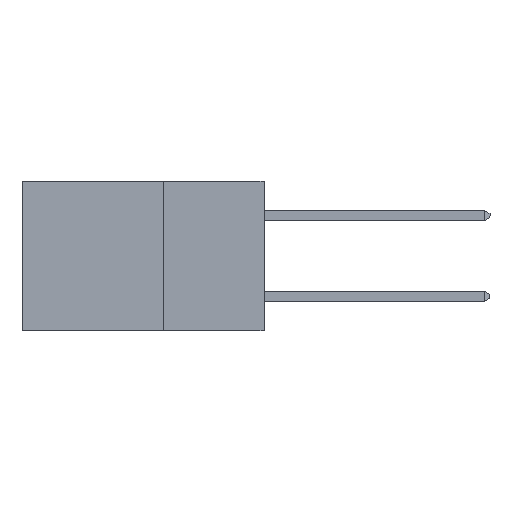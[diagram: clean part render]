
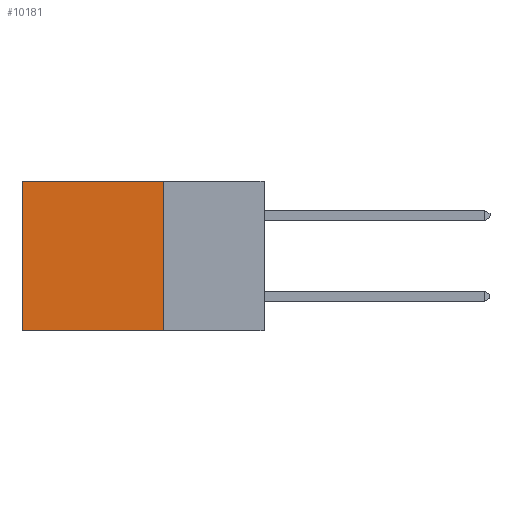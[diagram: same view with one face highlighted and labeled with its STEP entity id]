
A CAD part, left-side view. The second image highlights one B-rep face of the part: STEP entity #10181.
In plain terms, the highlighted planar face has unit normal (-1, 0, 0).
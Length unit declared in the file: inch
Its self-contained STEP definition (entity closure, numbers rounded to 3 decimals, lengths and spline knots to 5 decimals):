
#156 = CARTESIAN_POINT ( 'NONE',  ( 0.298, 0.25, 0. ) ) ;
#954 = VERTEX_POINT ( 'NONE', #5583 ) ;
#2154 = CARTESIAN_POINT ( 'NONE',  ( 0.298, 0.6, 0. ) ) ;
#3468 = EDGE_LOOP ( 'NONE', ( #4100, #5359, #7888, #10248 ) ) ;
#3909 = VERTEX_POINT ( 'NONE', #12758 ) ;
#4042 = DIRECTION ( 'NONE',  ( 1., 0., 0. ) ) ;
#4100 = ORIENTED_EDGE ( 'NONE', *, *, #11623, .T. ) ;
#4945 = DIRECTION ( 'NONE',  ( 0., 1., 0. ) ) ;
#4970 = VECTOR ( 'NONE', #4945, 39.37008 ) ;
#5121 = EDGE_CURVE ( 'NONE', #3909, #10668, #8246, .T. ) ;
#5158 = DIRECTION ( 'NONE',  ( 0., 1., 0. ) ) ;
#5359 = ORIENTED_EDGE ( 'NONE', *, *, #5121, .F. ) ;
#5583 = CARTESIAN_POINT ( 'NONE',  ( 0.298, 0.6, 0. ) ) ;
#5884 = VECTOR ( 'NONE', #11395, 39.37008 ) ;
#6391 = EDGE_CURVE ( 'NONE', #8597, #954, #7865, .T. ) ;
#7615 = VECTOR ( 'NONE', #7735, 39.37008 ) ;
#7735 = DIRECTION ( 'NONE',  ( 0., 0., -1. ) ) ;
#7865 = LINE ( 'NONE', #13925, #4970 ) ;
#7888 = ORIENTED_EDGE ( 'NONE', *, *, #13361, .F. ) ;
#8246 = LINE ( 'NONE', #9747, #13894 ) ;
#8597 = VERTEX_POINT ( 'NONE', #10443 ) ;
#9136 = CARTESIAN_POINT ( 'NONE',  ( 0.298, 0.6, -0.37 ) ) ;
#9747 = CARTESIAN_POINT ( 'NONE',  ( 0.298, 0.25, -0.37 ) ) ;
#10181 = ADVANCED_FACE ( 'NONE', ( #10243 ), #12959, .F. ) ;
#10243 = FACE_OUTER_BOUND ( 'NONE', #3468, .T. ) ;
#10248 = ORIENTED_EDGE ( 'NONE', *, *, #6391, .T. ) ;
#10443 = CARTESIAN_POINT ( 'NONE',  ( 0.298, 0.25, 0. ) ) ;
#10668 = VERTEX_POINT ( 'NONE', #9136 ) ;
#10696 = CARTESIAN_POINT ( 'NONE',  ( 0.298, 0.25, 0. ) ) ;
#11395 = DIRECTION ( 'NONE',  ( 0., 0., -1. ) ) ;
#11623 = EDGE_CURVE ( 'NONE', #954, #10668, #13630, .T. ) ;
#11885 = DIRECTION ( 'NONE',  ( 0., 0., -1. ) ) ;
#12758 = CARTESIAN_POINT ( 'NONE',  ( 0.298, 0.25, -0.37 ) ) ;
#12959 = PLANE ( 'NONE',  #14340 ) ;
#13361 = EDGE_CURVE ( 'NONE', #8597, #3909, #14061, .T. ) ;
#13630 = LINE ( 'NONE', #2154, #7615 ) ;
#13894 = VECTOR ( 'NONE', #5158, 39.37008 ) ;
#13925 = CARTESIAN_POINT ( 'NONE',  ( 0.298, 0.25, 0. ) ) ;
#14061 = LINE ( 'NONE', #156, #5884 ) ;
#14340 = AXIS2_PLACEMENT_3D ( 'NONE', #10696, #4042, #11885 ) ;
